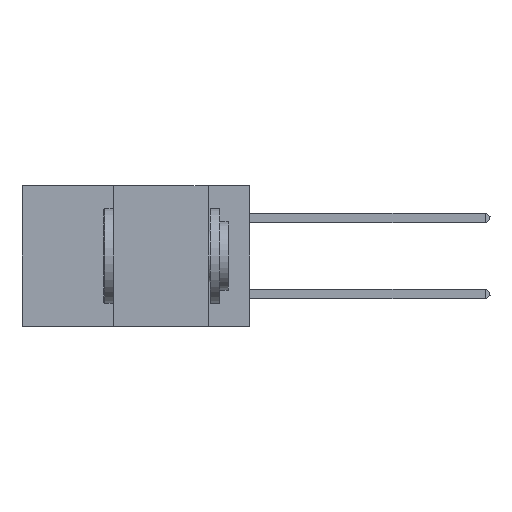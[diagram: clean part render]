
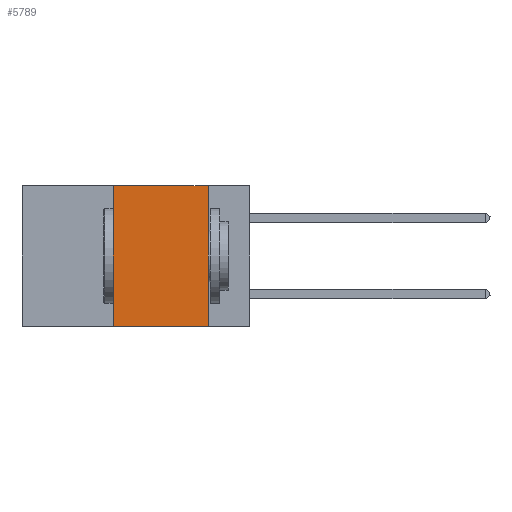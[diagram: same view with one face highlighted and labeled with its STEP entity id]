
A CAD part, left-side view. The second image highlights one B-rep face of the part: STEP entity #5789.
In plain terms, the highlighted planar face has unit normal (-1, 0, 0).
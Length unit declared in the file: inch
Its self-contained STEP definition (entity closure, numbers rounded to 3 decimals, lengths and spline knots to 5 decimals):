
#47 = ORIENTED_EDGE ( 'NONE', *, *, #8669, .F. ) ;
#183 = ORIENTED_EDGE ( 'NONE', *, *, #9576, .F. ) ;
#380 = ORIENTED_EDGE ( 'NONE', *, *, #8606, .T. ) ;
#393 = CARTESIAN_POINT ( 'NONE',  ( 0., 0.11, 0. ) ) ;
#658 = CARTESIAN_POINT ( 'NONE',  ( 0., 0.11, -0.37 ) ) ;
#769 = VECTOR ( 'NONE', #10906, 39.37008 ) ;
#1155 = LINE ( 'NONE', #6527, #3382 ) ;
#1469 = FACE_OUTER_BOUND ( 'NONE', #3907, .T. ) ;
#2211 = EDGE_CURVE ( 'NONE', #10116, #2608, #3313, .T. ) ;
#2529 = AXIS2_PLACEMENT_3D ( 'NONE', #9750, #9621, #9601 ) ;
#2608 = VERTEX_POINT ( 'NONE', #658 ) ;
#3032 = CARTESIAN_POINT ( 'NONE',  ( 0., 0.6, 0. ) ) ;
#3313 = LINE ( 'NONE', #393, #769 ) ;
#3382 = VECTOR ( 'NONE', #7435, 39.37008 ) ;
#3728 = CARTESIAN_POINT ( 'NONE',  ( 0., 0.11, 0. ) ) ;
#3907 = EDGE_LOOP ( 'NONE', ( #11190, #47, #183, #380 ) ) ;
#4379 = DIRECTION ( 'NONE',  ( 0., 0., 1. ) ) ;
#4652 = VECTOR ( 'NONE', #4379, 39.37008 ) ;
#4868 = DIRECTION ( 'NONE',  ( 0., -1., 0. ) ) ;
#5263 = CARTESIAN_POINT ( 'NONE',  ( 0., 0.36, 0. ) ) ;
#5789 = ADVANCED_FACE ( 'NONE', ( #1469 ), #9644, .F. ) ;
#6026 = VERTEX_POINT ( 'NONE', #8113 ) ;
#6527 = CARTESIAN_POINT ( 'NONE',  ( 0., 0.6, -0.37 ) ) ;
#6962 = LINE ( 'NONE', #5263, #4652 ) ;
#7123 = CARTESIAN_POINT ( 'NONE',  ( 0., 0.36, 0. ) ) ;
#7267 = VECTOR ( 'NONE', #4868, 39.37008 ) ;
#7435 = DIRECTION ( 'NONE',  ( 0., -1., 0. ) ) ;
#7708 = VERTEX_POINT ( 'NONE', #7123 ) ;
#8113 = CARTESIAN_POINT ( 'NONE',  ( 0., 0.36, -0.37 ) ) ;
#8606 = EDGE_CURVE ( 'NONE', #6026, #2608, #1155, .T. ) ;
#8669 = EDGE_CURVE ( 'NONE', #7708, #10116, #9563, .T. ) ;
#9563 = LINE ( 'NONE', #3032, #7267 ) ;
#9576 = EDGE_CURVE ( 'NONE', #6026, #7708, #6962, .T. ) ;
#9601 = DIRECTION ( 'NONE',  ( 0., 0., -1. ) ) ;
#9621 = DIRECTION ( 'NONE',  ( 1., 0., 0. ) ) ;
#9644 = PLANE ( 'NONE',  #2529 ) ;
#9750 = CARTESIAN_POINT ( 'NONE',  ( 0., 0.6, 0. ) ) ;
#10116 = VERTEX_POINT ( 'NONE', #3728 ) ;
#10906 = DIRECTION ( 'NONE',  ( 0., 0., -1. ) ) ;
#11190 = ORIENTED_EDGE ( 'NONE', *, *, #2211, .F. ) ;
